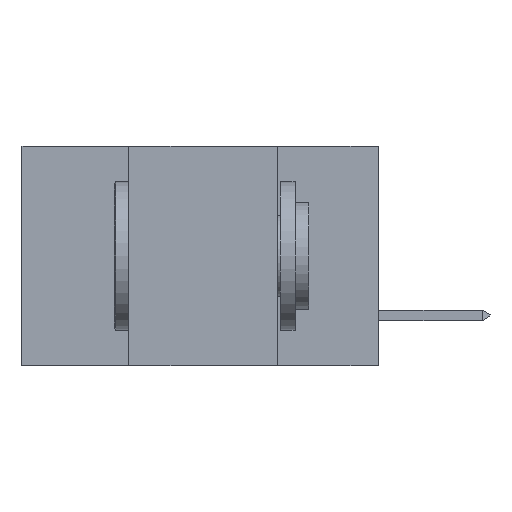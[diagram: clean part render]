
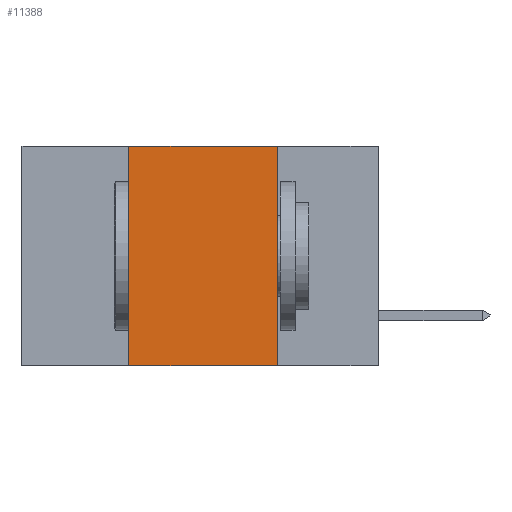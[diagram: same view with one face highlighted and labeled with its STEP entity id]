
A CAD part, left-side view. The second image highlights one B-rep face of the part: STEP entity #11388.
In plain terms, the highlighted planar face has unit normal (-1, 0, 0).
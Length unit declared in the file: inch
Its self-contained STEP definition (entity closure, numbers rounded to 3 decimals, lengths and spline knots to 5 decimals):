
#706 = AXIS2_PLACEMENT_3D ( 'NONE', #29749, #32313, #19681 ) ;
#2721 = FACE_OUTER_BOUND ( 'NONE', #29468, .T. ) ;
#3440 = EDGE_CURVE ( 'NONE', #21114, #13514, #27454, .T. ) ;
#3538 = LINE ( 'NONE', #4797, #29594 ) ;
#4120 = VERTEX_POINT ( 'NONE', #22141 ) ;
#4432 = LINE ( 'NONE', #27442, #16209 ) ;
#4546 = CARTESIAN_POINT ( 'NONE',  ( 0., 0.42, -0.37 ) ) ;
#4684 = DIRECTION ( 'NONE',  ( 0., -1., 0. ) ) ;
#4797 = CARTESIAN_POINT ( 'NONE',  ( 0., 0.6, 0. ) ) ;
#5596 = VECTOR ( 'NONE', #4684, 39.37008 ) ;
#6985 = EDGE_CURVE ( 'NONE', #4120, #21114, #3538, .T. ) ;
#7175 = ORIENTED_EDGE ( 'NONE', *, *, #6985, .F. ) ;
#7360 = DIRECTION ( 'NONE',  ( 0., -1., 0. ) ) ;
#8419 = ORIENTED_EDGE ( 'NONE', *, *, #3440, .F. ) ;
#11388 = ADVANCED_FACE ( 'NONE', ( #2721 ), #27239, .F. ) ;
#13514 = VERTEX_POINT ( 'NONE', #14012 ) ;
#14012 = CARTESIAN_POINT ( 'NONE',  ( 0., 0.17, -0.37 ) ) ;
#14391 = DIRECTION ( 'NONE',  ( 0., 0., 1. ) ) ;
#15263 = EDGE_CURVE ( 'NONE', #23718, #13514, #23334, .T. ) ;
#15455 = ORIENTED_EDGE ( 'NONE', *, *, #15263, .T. ) ;
#16209 = VECTOR ( 'NONE', #14391, 39.37008 ) ;
#18943 = ORIENTED_EDGE ( 'NONE', *, *, #22758, .F. ) ;
#19217 = CARTESIAN_POINT ( 'NONE',  ( 0., 0.17, 0. ) ) ;
#19681 = DIRECTION ( 'NONE',  ( 0., 0., -1. ) ) ;
#19759 = CARTESIAN_POINT ( 'NONE',  ( 0., 0.6, -0.37 ) ) ;
#21114 = VERTEX_POINT ( 'NONE', #23411 ) ;
#22109 = DIRECTION ( 'NONE',  ( 0., 0., -1. ) ) ;
#22141 = CARTESIAN_POINT ( 'NONE',  ( 0., 0.42, 0. ) ) ;
#22758 = EDGE_CURVE ( 'NONE', #23718, #4120, #4432, .T. ) ;
#23334 = LINE ( 'NONE', #19759, #5596 ) ;
#23411 = CARTESIAN_POINT ( 'NONE',  ( 0., 0.17, 0. ) ) ;
#23718 = VERTEX_POINT ( 'NONE', #4546 ) ;
#27239 = PLANE ( 'NONE',  #706 ) ;
#27442 = CARTESIAN_POINT ( 'NONE',  ( 0., 0.42, 0. ) ) ;
#27454 = LINE ( 'NONE', #19217, #28642 ) ;
#28642 = VECTOR ( 'NONE', #22109, 39.37008 ) ;
#29468 = EDGE_LOOP ( 'NONE', ( #8419, #7175, #18943, #15455 ) ) ;
#29594 = VECTOR ( 'NONE', #7360, 39.37008 ) ;
#29749 = CARTESIAN_POINT ( 'NONE',  ( 0., 0.6, 0. ) ) ;
#32313 = DIRECTION ( 'NONE',  ( 1., 0., 0. ) ) ;
